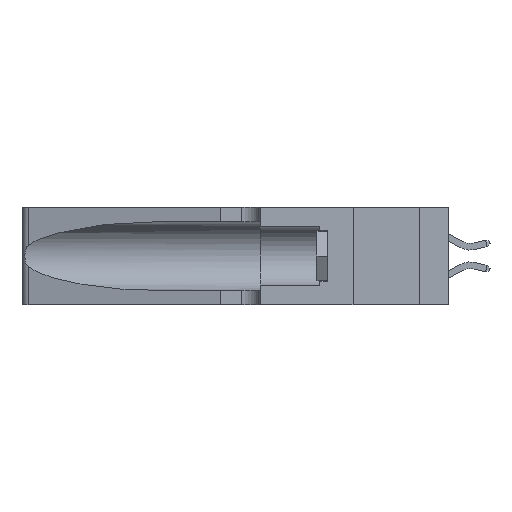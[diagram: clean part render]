
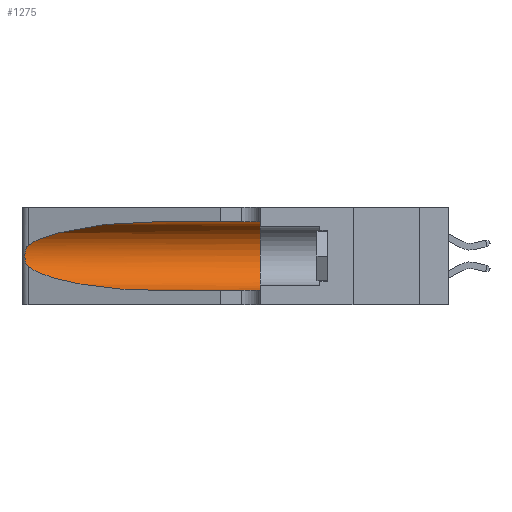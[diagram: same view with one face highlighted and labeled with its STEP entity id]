
A CAD part, left-side view. The second image highlights one B-rep face of the part: STEP entity #1275.
In plain terms, the highlighted cylindrical face has radius 3.308 mm (diameter 6.617 mm), a partial arc.
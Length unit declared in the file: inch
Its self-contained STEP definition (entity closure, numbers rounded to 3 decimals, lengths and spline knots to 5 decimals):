
#62 = DIRECTION ( 'NONE',  ( 0., 0., 1. ) ) ;
#326 = CARTESIAN_POINT ( 'NONE',  ( 0.2373, 1.15595, 0.28018 ) ) ;
#356 = AXIS2_PLACEMENT_3D ( 'NONE', #1134, #6045, #9468 ) ;
#1134 = CARTESIAN_POINT ( 'NONE',  ( 0.1305, 1.61858, 0.185 ) ) ;
#1275 = ADVANCED_FACE ( 'NONE', ( #16411 ), #4672, .F. ) ;
#1431 = CARTESIAN_POINT ( 'NONE',  ( 0.1305, 0.35, 0.185 ) ) ;
#1523 = CARTESIAN_POINT ( 'NONE',  ( 0.25487, 1.22718, 0.14631 ) ) ;
#1709 = VECTOR ( 'NONE', #3958, 39.37008 ) ;
#2048 = CARTESIAN_POINT ( 'NONE',  ( 0.26075, 1.23896, 0.178 ) ) ;
#2896 = EDGE_LOOP ( 'NONE', ( #18102, #11776, #18693, #10841, #3324, #9052 ) ) ;
#3324 = ORIENTED_EDGE ( 'NONE', *, *, #15214, .F. ) ;
#3370 =( BOUNDED_CURVE ( )  B_SPLINE_CURVE ( 3, ( #6228, #4526, #3947, #18582 ),
 .UNSPECIFIED., .F., .F. ) 
 B_SPLINE_CURVE_WITH_KNOTS ( ( 4, 4 ),
 ( 3.44316, 4.71239 ),
 .UNSPECIFIED. ) 
 CURVE ( )  GEOMETRIC_REPRESENTATION_ITEM ( )  RATIONAL_B_SPLINE_CURVE ( ( 1., 0.87, 0.87, 1. ) ) 
 REPRESENTATION_ITEM ( '' )  );
#3812 = CARTESIAN_POINT ( 'NONE',  ( 0.1305, 1.61858, 0.31525 ) ) ;
#3947 = CARTESIAN_POINT ( 'NONE',  ( 0.18966, 0.96281, 0.05475 ) ) ;
#3958 = DIRECTION ( 'NONE',  ( 0., -1., 0. ) ) ;
#4014 = CARTESIAN_POINT ( 'NONE',  ( 0.26075, 1.23896, 0.19203 ) ) ;
#4323 = CARTESIAN_POINT ( 'NONE',  ( 0.1305, 0.72297, 0.05475 ) ) ;
#4526 = CARTESIAN_POINT ( 'NONE',  ( 0.2373, 1.15595, 0.08982 ) ) ;
#4666 = EDGE_CURVE ( 'NONE', #8955, #8083, #6768, .T. ) ;
#4672 = CYLINDRICAL_SURFACE ( 'NONE', #356, 0.13025 ) ;
#5276 = EDGE_CURVE ( 'NONE', #9820, #10501, #9683, .T. ) ;
#5522 = CARTESIAN_POINT ( 'NONE',  ( 0.25854, 1.2359, 0.20912 ) ) ;
#5533 = CIRCLE ( 'NONE', #19787, 0.13025 ) ;
#5587 = CARTESIAN_POINT ( 'NONE',  ( 0.25555, 1.22994, 0.2215 ) ) ;
#6045 = DIRECTION ( 'NONE',  ( 0., -1., 0. ) ) ;
#6228 = CARTESIAN_POINT ( 'NONE',  ( 0.25487, 1.22718, 0.14631 ) ) ;
#6498 = EDGE_CURVE ( 'NONE', #19476, #9820, #3370, .T. ) ;
#6768 =( BOUNDED_CURVE ( )  B_SPLINE_CURVE ( 3, ( #20199, #10442, #326, #13575 ),
 .UNSPECIFIED., .F., .T. ) 
 B_SPLINE_CURVE_WITH_KNOTS ( ( 4, 4 ),
 ( 1.5708, 2.84003 ),
 .UNSPECIFIED. ) 
 CURVE ( )  GEOMETRIC_REPRESENTATION_ITEM ( )  RATIONAL_B_SPLINE_CURVE ( ( 1., 0.87, 0.87, 1. ) ) 
 REPRESENTATION_ITEM ( '' )  );
#7062 = CARTESIAN_POINT ( 'NONE',  ( 0.25487, 1.22718, 0.22369 ) ) ;
#7134 = CARTESIAN_POINT ( 'NONE',  ( 0.25639, 1.23184, 0.21858 ) ) ;
#7277 = DIRECTION ( 'NONE',  ( 0., -1., 0. ) ) ;
#8083 = VERTEX_POINT ( 'NONE', #11044 ) ;
#8632 = CARTESIAN_POINT ( 'NONE',  ( 0.25555, 1.22993, 0.14849 ) ) ;
#8704 = CARTESIAN_POINT ( 'NONE',  ( 0.26017, 1.23833, 0.17102 ) ) ;
#8783 = CARTESIAN_POINT ( 'NONE',  ( 0.25789, 1.23486, 0.15765 ) ) ;
#8955 = VERTEX_POINT ( 'NONE', #12368 ) ;
#9052 = ORIENTED_EDGE ( 'NONE', *, *, #13930, .F. ) ;
#9468 = DIRECTION ( 'NONE',  ( 0., 0., -1. ) ) ;
#9683 = LINE ( 'NONE', #10296, #20109 ) ;
#9820 = VERTEX_POINT ( 'NONE', #4323 ) ;
#10296 = CARTESIAN_POINT ( 'NONE',  ( 0.1305, 1.61858, 0.05475 ) ) ;
#10442 = CARTESIAN_POINT ( 'NONE',  ( 0.18966, 0.96281, 0.31525 ) ) ;
#10501 = VERTEX_POINT ( 'NONE', #12637 ) ;
#10841 = ORIENTED_EDGE ( 'NONE', *, *, #5276, .T. ) ;
#11044 = CARTESIAN_POINT ( 'NONE',  ( 0.25487, 1.22718, 0.22369 ) ) ;
#11776 = ORIENTED_EDGE ( 'NONE', *, *, #13122, .T. ) ;
#12008 = CARTESIAN_POINT ( 'NONE',  ( 0.26018, 1.23835, 0.19895 ) ) ;
#12084 = CARTESIAN_POINT ( 'NONE',  ( 0.25639, 1.23186, 0.15144 ) ) ;
#12368 = CARTESIAN_POINT ( 'NONE',  ( 0.1305, 0.72297, 0.31525 ) ) ;
#12637 = CARTESIAN_POINT ( 'NONE',  ( 0.1305, 0.35, 0.05475 ) ) ;
#13122 = EDGE_CURVE ( 'NONE', #8083, #19476, #20766, .T. ) ;
#13575 = CARTESIAN_POINT ( 'NONE',  ( 0.25487, 1.22718, 0.22369 ) ) ;
#13699 = CARTESIAN_POINT ( 'NONE',  ( 0.25487, 1.22718, 0.14631 ) ) ;
#13930 = EDGE_CURVE ( 'NONE', #8955, #20612, #18590, .T. ) ;
#14279 = CARTESIAN_POINT ( 'NONE',  ( 0.1305, 0.35, 0.31525 ) ) ;
#15214 = EDGE_CURVE ( 'NONE', #20612, #10501, #5533, .T. ) ;
#16411 = FACE_OUTER_BOUND ( 'NONE', #2896, .T. ) ;
#16924 = CARTESIAN_POINT ( 'NONE',  ( 0.25856, 1.23593, 0.16098 ) ) ;
#17808 = DIRECTION ( 'NONE',  ( 0., 1., 0. ) ) ;
#18102 = ORIENTED_EDGE ( 'NONE', *, *, #4666, .T. ) ;
#18411 = CARTESIAN_POINT ( 'NONE',  ( 0.25787, 1.23484, 0.2124 ) ) ;
#18582 = CARTESIAN_POINT ( 'NONE',  ( 0.1305, 0.72297, 0.05475 ) ) ;
#18590 = LINE ( 'NONE', #3812, #1709 ) ;
#18693 = ORIENTED_EDGE ( 'NONE', *, *, #6498, .T. ) ;
#19476 = VERTEX_POINT ( 'NONE', #1523 ) ;
#19787 = AXIS2_PLACEMENT_3D ( 'NONE', #1431, #17808, #62 ) ;
#20109 = VECTOR ( 'NONE', #7277, 39.37008 ) ;
#20199 = CARTESIAN_POINT ( 'NONE',  ( 0.1305, 0.72297, 0.31525 ) ) ;
#20612 = VERTEX_POINT ( 'NONE', #14279 ) ;
#20766 = B_SPLINE_CURVE_WITH_KNOTS ( 'NONE', 3,
 ( #7062, #5587, #7134, #18411, #5522, #12008, #4014, #2048, #8704, #16924, #8783, #12084, #8632, #13699 ),
 .UNSPECIFIED., .F., .F.,
 ( 4, 2, 2, 2, 2, 2, 4 ),
 ( 0., 0.00027, 0.00053, 0.00107, 0.0016, 0.00187, 0.00214 ),
 .UNSPECIFIED. ) ;
